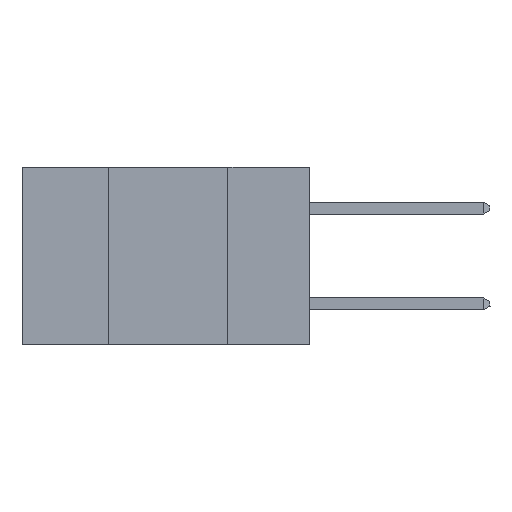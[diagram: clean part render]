
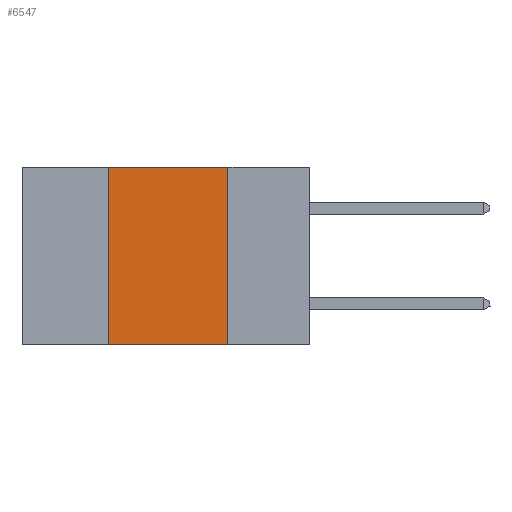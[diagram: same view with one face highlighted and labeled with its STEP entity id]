
A CAD part, left-side view. The second image highlights one B-rep face of the part: STEP entity #6547.
In plain terms, the highlighted planar face has unit normal (-1, 0, 0).
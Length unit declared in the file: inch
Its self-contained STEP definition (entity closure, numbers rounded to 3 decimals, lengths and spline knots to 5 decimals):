
#2021 = VECTOR ( 'NONE', #2850, 39.37008 ) ;
#2258 = CARTESIAN_POINT ( 'NONE',  ( 0., 0.17, 0. ) ) ;
#2655 = ORIENTED_EDGE ( 'NONE', *, *, #15043, .F. ) ;
#2850 = DIRECTION ( 'NONE',  ( 0., -1., 0. ) ) ;
#2870 = CARTESIAN_POINT ( 'NONE',  ( 0., 0.6, 0. ) ) ;
#3855 = ORIENTED_EDGE ( 'NONE', *, *, #11975, .T. ) ;
#4052 = VERTEX_POINT ( 'NONE', #5223 ) ;
#4402 = DIRECTION ( 'NONE',  ( 0., -1., 0. ) ) ;
#5223 = CARTESIAN_POINT ( 'NONE',  ( 0., 0.42, -0.37 ) ) ;
#5376 = CARTESIAN_POINT ( 'NONE',  ( 0., 0.42, 0. ) ) ;
#6053 = VECTOR ( 'NONE', #7995, 39.37008 ) ;
#6094 = FACE_OUTER_BOUND ( 'NONE', #11299, .T. ) ;
#6205 = DIRECTION ( 'NONE',  ( 1., 0., 0. ) ) ;
#6547 = ADVANCED_FACE ( 'NONE', ( #6094 ), #14867, .F. ) ;
#6650 = CARTESIAN_POINT ( 'NONE',  ( 0., 0.17, 0. ) ) ;
#6778 = EDGE_CURVE ( 'NONE', #18461, #14096, #10296, .T. ) ;
#7423 = EDGE_CURVE ( 'NONE', #4052, #10506, #13772, .T. ) ;
#7995 = DIRECTION ( 'NONE',  ( 0., 0., 1. ) ) ;
#8822 = VECTOR ( 'NONE', #4402, 39.37008 ) ;
#9259 = ORIENTED_EDGE ( 'NONE', *, *, #6778, .F. ) ;
#9754 = LINE ( 'NONE', #2870, #8822 ) ;
#9776 = CARTESIAN_POINT ( 'NONE',  ( 0., 0.17, -0.37 ) ) ;
#10296 = LINE ( 'NONE', #6650, #12732 ) ;
#10506 = VERTEX_POINT ( 'NONE', #5376 ) ;
#11299 = EDGE_LOOP ( 'NONE', ( #9259, #2655, #18274, #3855 ) ) ;
#11975 = EDGE_CURVE ( 'NONE', #4052, #14096, #14713, .T. ) ;
#12070 = CARTESIAN_POINT ( 'NONE',  ( 0., 0.6, 0. ) ) ;
#12544 = DIRECTION ( 'NONE',  ( 0., 0., -1. ) ) ;
#12732 = VECTOR ( 'NONE', #12544, 39.37008 ) ;
#13194 = CARTESIAN_POINT ( 'NONE',  ( 0., 0.6, -0.37 ) ) ;
#13772 = LINE ( 'NONE', #15132, #6053 ) ;
#14091 = AXIS2_PLACEMENT_3D ( 'NONE', #12070, #6205, #16230 ) ;
#14096 = VERTEX_POINT ( 'NONE', #9776 ) ;
#14713 = LINE ( 'NONE', #13194, #2021 ) ;
#14867 = PLANE ( 'NONE',  #14091 ) ;
#15043 = EDGE_CURVE ( 'NONE', #10506, #18461, #9754, .T. ) ;
#15132 = CARTESIAN_POINT ( 'NONE',  ( 0., 0.42, 0. ) ) ;
#16230 = DIRECTION ( 'NONE',  ( 0., 0., -1. ) ) ;
#18274 = ORIENTED_EDGE ( 'NONE', *, *, #7423, .F. ) ;
#18461 = VERTEX_POINT ( 'NONE', #2258 ) ;
